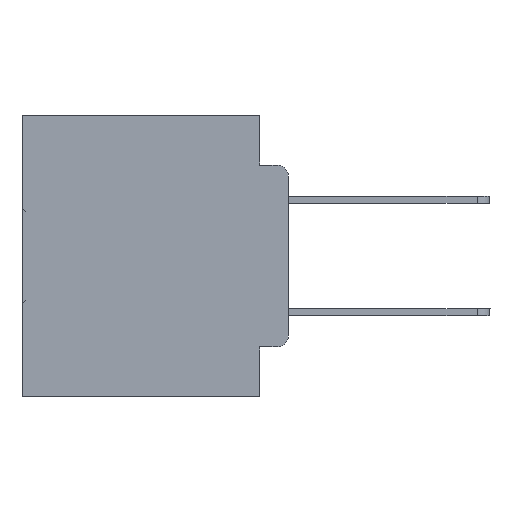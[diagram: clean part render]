
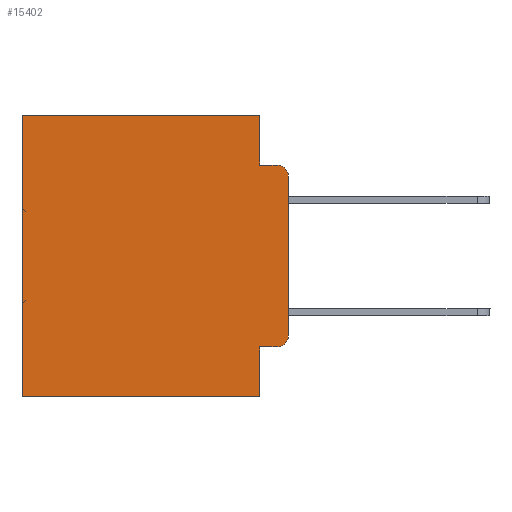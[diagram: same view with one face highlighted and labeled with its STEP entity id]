
A CAD part, left-side view. The second image highlights one B-rep face of the part: STEP entity #15402.
In plain terms, the highlighted planar face has unit normal (-1, 0, 0).
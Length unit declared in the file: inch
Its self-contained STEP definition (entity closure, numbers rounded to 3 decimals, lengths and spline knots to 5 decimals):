
#1827 = ORIENTED_EDGE ( 'NONE', *, *, #23706, .T. ) ;
#1935 = DIRECTION ( 'NONE',  ( 0., -1., 0. ) ) ;
#2060 = LINE ( 'NONE', #11316, #7805 ) ;
#2259 = ORIENTED_EDGE ( 'NONE', *, *, #30628, .T. ) ;
#3654 = CARTESIAN_POINT ( 'NONE',  ( 0.298, 0., 0. ) ) ;
#3952 = CARTESIAN_POINT ( 'NONE',  ( 0.298, 0., -0.1085 ) ) ;
#4031 = VERTEX_POINT ( 'NONE', #9395 ) ;
#4156 = LINE ( 'NONE', #5787, #5057 ) ;
#4208 = CARTESIAN_POINT ( 'NONE',  ( 0.298, 0.02, -0.1085 ) ) ;
#4929 = ORIENTED_EDGE ( 'NONE', *, *, #23539, .T. ) ;
#5057 = VECTOR ( 'NONE', #22629, 39.37008 ) ;
#5109 = CARTESIAN_POINT ( 'NONE',  ( 0.298, 0.473, 0. ) ) ;
#5787 = CARTESIAN_POINT ( 'NONE',  ( 0.298, 0.051, 0. ) ) ;
#6128 = VERTEX_POINT ( 'NONE', #17095 ) ;
#6302 = CARTESIAN_POINT ( 'NONE',  ( 0.298, 0.051, 0. ) ) ;
#6829 = EDGE_LOOP ( 'NONE', ( #10673, #2259, #26413, #18182, #12435, #4929, #29019, #28144, #16860, #1827 ) ) ;
#7069 = DIRECTION ( 'NONE',  ( 0., 0., -1. ) ) ;
#7805 = VECTOR ( 'NONE', #22510, 39.37008 ) ;
#8458 = PLANE ( 'NONE',  #14340 ) ;
#8585 = VERTEX_POINT ( 'NONE', #11007 ) ;
#8787 = CARTESIAN_POINT ( 'NONE',  ( 0.298, 0.02, -0.3915 ) ) ;
#9053 = VECTOR ( 'NONE', #1935, 39.37008 ) ;
#9113 = VECTOR ( 'NONE', #19692, 39.37008 ) ;
#9395 = CARTESIAN_POINT ( 'NONE',  ( 0.298, 0.051, -0.4115 ) ) ;
#9553 = CIRCLE ( 'NONE', #23126, 0.02 ) ;
#10581 = EDGE_CURVE ( 'NONE', #13332, #19047, #32368, .T. ) ;
#10673 = ORIENTED_EDGE ( 'NONE', *, *, #10581, .F. ) ;
#10822 = VERTEX_POINT ( 'NONE', #23824 ) ;
#11007 = CARTESIAN_POINT ( 'NONE',  ( 0.298, 0.473, 0. ) ) ;
#11291 = DIRECTION ( 'NONE',  ( 1., 0., 0. ) ) ;
#11316 = CARTESIAN_POINT ( 'NONE',  ( 0.298, 0.051, 0. ) ) ;
#11408 = CARTESIAN_POINT ( 'NONE',  ( 0.298, 0.02, -0.0885 ) ) ;
#11462 = VERTEX_POINT ( 'NONE', #21506 ) ;
#11645 = DIRECTION ( 'NONE',  ( 0., 0., -1. ) ) ;
#12435 = ORIENTED_EDGE ( 'NONE', *, *, #29889, .T. ) ;
#12875 = AXIS2_PLACEMENT_3D ( 'NONE', #8787, #28342, #11645 ) ;
#13332 = VERTEX_POINT ( 'NONE', #3952 ) ;
#13379 = CARTESIAN_POINT ( 'NONE',  ( 0.298, 0., -0.5 ) ) ;
#14340 = AXIS2_PLACEMENT_3D ( 'NONE', #33490, #11291, #30814 ) ;
#15266 = VECTOR ( 'NONE', #16242, 39.37008 ) ;
#15402 = ADVANCED_FACE ( 'NONE', ( #19930 ), #8458, .F. ) ;
#15899 = LINE ( 'NONE', #5109, #33284 ) ;
#16242 = DIRECTION ( 'NONE',  ( 0., 1., 0. ) ) ;
#16860 = ORIENTED_EDGE ( 'NONE', *, *, #19169, .T. ) ;
#17095 = CARTESIAN_POINT ( 'NONE',  ( 0.298, 0.473, -0.5 ) ) ;
#18182 = ORIENTED_EDGE ( 'NONE', *, *, #29520, .F. ) ;
#18491 = VECTOR ( 'NONE', #30978, 39.37008 ) ;
#19047 = VERTEX_POINT ( 'NONE', #29270 ) ;
#19169 = EDGE_CURVE ( 'NONE', #4031, #10822, #24836, .T. ) ;
#19312 = VECTOR ( 'NONE', #20562, 39.37008 ) ;
#19692 = DIRECTION ( 'NONE',  ( 0., -1., 0. ) ) ;
#19930 = FACE_OUTER_BOUND ( 'NONE', #6829, .T. ) ;
#19951 = CARTESIAN_POINT ( 'NONE',  ( 0.298, 0., 0. ) ) ;
#20562 = DIRECTION ( 'NONE',  ( 0., 1., 0. ) ) ;
#21506 = CARTESIAN_POINT ( 'NONE',  ( 0.298, 0.051, -0.5 ) ) ;
#21977 = DIRECTION ( 'NONE',  ( 0., 0., -1. ) ) ;
#22510 = DIRECTION ( 'NONE',  ( 0., 0., -1. ) ) ;
#22629 = DIRECTION ( 'NONE',  ( 0., 0., -1. ) ) ;
#23126 = AXIS2_PLACEMENT_3D ( 'NONE', #4208, #23889, #7069 ) ;
#23539 = EDGE_CURVE ( 'NONE', #8585, #6128, #15899, .T. ) ;
#23706 = EDGE_CURVE ( 'NONE', #10822, #19047, #31081, .T. ) ;
#23824 = CARTESIAN_POINT ( 'NONE',  ( 0.298, 0.02, -0.4115 ) ) ;
#23889 = DIRECTION ( 'NONE',  ( -1., 0., 0. ) ) ;
#24836 = LINE ( 'NONE', #35484, #9053 ) ;
#25143 = CARTESIAN_POINT ( 'NONE',  ( 0.298, 0.051, -0.0885 ) ) ;
#25273 = LINE ( 'NONE', #13379, #15266 ) ;
#26074 = EDGE_CURVE ( 'NONE', #11462, #6128, #25273, .T. ) ;
#26413 = ORIENTED_EDGE ( 'NONE', *, *, #29687, .F. ) ;
#28144 = ORIENTED_EDGE ( 'NONE', *, *, #31649, .F. ) ;
#28342 = DIRECTION ( 'NONE',  ( -1., 0., 0. ) ) ;
#29019 = ORIENTED_EDGE ( 'NONE', *, *, #26074, .F. ) ;
#29270 = CARTESIAN_POINT ( 'NONE',  ( 0.298, 0., -0.3915 ) ) ;
#29520 = EDGE_CURVE ( 'NONE', #33417, #35633, #2060, .T. ) ;
#29687 = EDGE_CURVE ( 'NONE', #35633, #30347, #33148, .T. ) ;
#29889 = EDGE_CURVE ( 'NONE', #33417, #8585, #34063, .T. ) ;
#30347 = VERTEX_POINT ( 'NONE', #11408 ) ;
#30628 = EDGE_CURVE ( 'NONE', #13332, #30347, #9553, .T. ) ;
#30814 = DIRECTION ( 'NONE',  ( 0., 0., -1. ) ) ;
#30978 = DIRECTION ( 'NONE',  ( 0., 0., -1. ) ) ;
#31081 = CIRCLE ( 'NONE', #12875, 0.02 ) ;
#31151 = CARTESIAN_POINT ( 'NONE',  ( 0.298, 0.051, -0.0885 ) ) ;
#31649 = EDGE_CURVE ( 'NONE', #4031, #11462, #4156, .T. ) ;
#32368 = LINE ( 'NONE', #19951, #18491 ) ;
#33148 = LINE ( 'NONE', #25143, #9113 ) ;
#33284 = VECTOR ( 'NONE', #21977, 39.37008 ) ;
#33417 = VERTEX_POINT ( 'NONE', #6302 ) ;
#33490 = CARTESIAN_POINT ( 'NONE',  ( 0.298, 0., 0. ) ) ;
#34063 = LINE ( 'NONE', #3654, #19312 ) ;
#35484 = CARTESIAN_POINT ( 'NONE',  ( 0.298, 0.051, -0.4115 ) ) ;
#35633 = VERTEX_POINT ( 'NONE', #31151 ) ;
